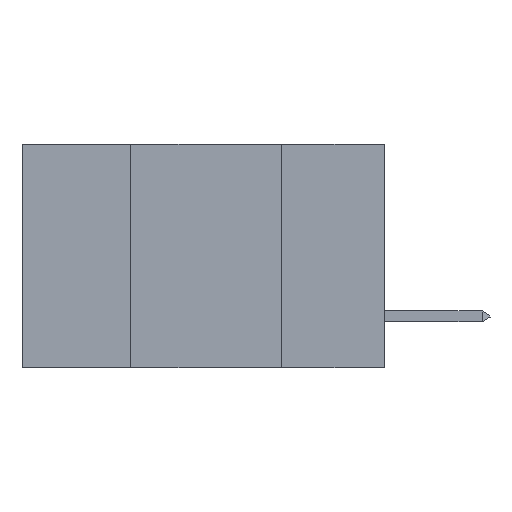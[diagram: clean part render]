
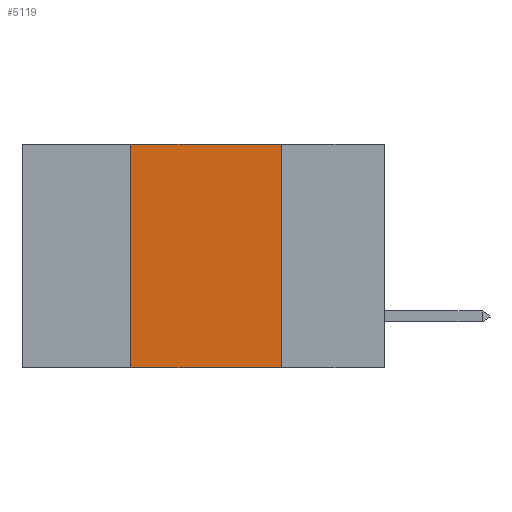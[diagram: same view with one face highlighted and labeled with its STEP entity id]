
A CAD part, left-side view. The second image highlights one B-rep face of the part: STEP entity #5119.
In plain terms, the highlighted planar face has unit normal (-1, 0, 0).
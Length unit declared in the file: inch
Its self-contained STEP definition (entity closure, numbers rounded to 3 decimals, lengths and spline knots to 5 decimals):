
#37 = VERTEX_POINT ( 'NONE', #2293 ) ;
#641 = ORIENTED_EDGE ( 'NONE', *, *, #5775, .T. ) ;
#1115 = CARTESIAN_POINT ( 'NONE',  ( 0., 0.6, -0.37 ) ) ;
#2293 = CARTESIAN_POINT ( 'NONE',  ( 0., 0.42, -0.37 ) ) ;
#2671 = VECTOR ( 'NONE', #4944, 39.37008 ) ;
#2727 = VERTEX_POINT ( 'NONE', #12356 ) ;
#4173 = LINE ( 'NONE', #7064, #7596 ) ;
#4391 = VECTOR ( 'NONE', #10264, 39.37008 ) ;
#4775 = ORIENTED_EDGE ( 'NONE', *, *, #5073, .F. ) ;
#4944 = DIRECTION ( 'NONE',  ( 0., -1., 0. ) ) ;
#5073 = EDGE_CURVE ( 'NONE', #37, #2727, #8600, .T. ) ;
#5119 = ADVANCED_FACE ( 'NONE', ( #14353 ), #5491, .F. ) ;
#5382 = CARTESIAN_POINT ( 'NONE',  ( 0., 0.6, 0. ) ) ;
#5491 = PLANE ( 'NONE',  #9426 ) ;
#5775 = EDGE_CURVE ( 'NONE', #37, #13522, #13389, .T. ) ;
#6487 = CARTESIAN_POINT ( 'NONE',  ( 0., 0.17, 0. ) ) ;
#6631 = EDGE_CURVE ( 'NONE', #7308, #13522, #4173, .T. ) ;
#7064 = CARTESIAN_POINT ( 'NONE',  ( 0., 0.17, 0. ) ) ;
#7308 = VERTEX_POINT ( 'NONE', #6487 ) ;
#7596 = VECTOR ( 'NONE', #13233, 39.37008 ) ;
#7691 = EDGE_LOOP ( 'NONE', ( #13113, #10703, #4775, #641 ) ) ;
#7818 = DIRECTION ( 'NONE',  ( 1., 0., 0. ) ) ;
#8026 = CARTESIAN_POINT ( 'NONE',  ( 0., 0.42, 0. ) ) ;
#8199 = CARTESIAN_POINT ( 'NONE',  ( 0., 0.17, -0.37 ) ) ;
#8600 = LINE ( 'NONE', #8026, #14179 ) ;
#9426 = AXIS2_PLACEMENT_3D ( 'NONE', #5382, #7818, #11539 ) ;
#10093 = CARTESIAN_POINT ( 'NONE',  ( 0., 0.6, 0. ) ) ;
#10264 = DIRECTION ( 'NONE',  ( 0., -1., 0. ) ) ;
#10703 = ORIENTED_EDGE ( 'NONE', *, *, #12091, .F. ) ;
#11539 = DIRECTION ( 'NONE',  ( 0., 0., -1. ) ) ;
#12091 = EDGE_CURVE ( 'NONE', #2727, #7308, #14704, .T. ) ;
#12356 = CARTESIAN_POINT ( 'NONE',  ( 0., 0.42, 0. ) ) ;
#13113 = ORIENTED_EDGE ( 'NONE', *, *, #6631, .F. ) ;
#13233 = DIRECTION ( 'NONE',  ( 0., 0., -1. ) ) ;
#13389 = LINE ( 'NONE', #1115, #2671 ) ;
#13522 = VERTEX_POINT ( 'NONE', #8199 ) ;
#14160 = DIRECTION ( 'NONE',  ( 0., 0., 1. ) ) ;
#14179 = VECTOR ( 'NONE', #14160, 39.37008 ) ;
#14353 = FACE_OUTER_BOUND ( 'NONE', #7691, .T. ) ;
#14704 = LINE ( 'NONE', #10093, #4391 ) ;
